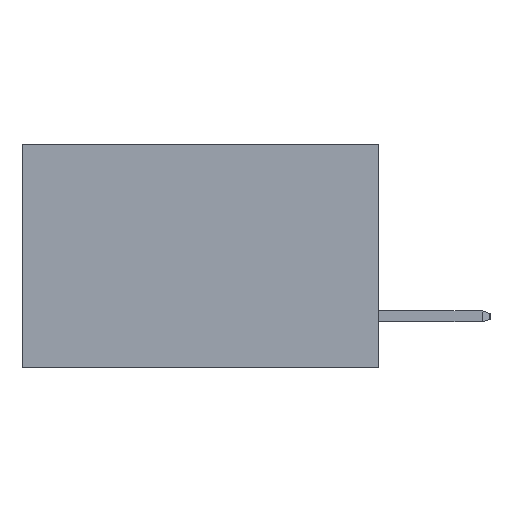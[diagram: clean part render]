
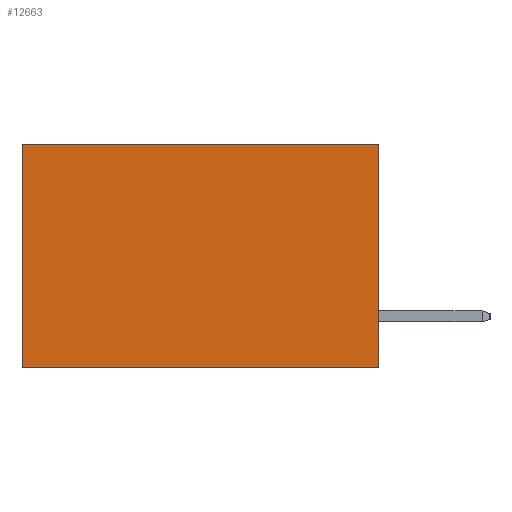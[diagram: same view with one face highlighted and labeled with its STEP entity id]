
A CAD part, left-side view. The second image highlights one B-rep face of the part: STEP entity #12663.
In plain terms, the highlighted planar face has unit normal (-1, 0, 0).
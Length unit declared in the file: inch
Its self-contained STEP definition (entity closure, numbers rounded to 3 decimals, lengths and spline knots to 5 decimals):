
#49 = CARTESIAN_POINT ( 'NONE',  ( 0.277, 0., -0.37 ) ) ;
#526 = LINE ( 'NONE', #4320, #6119 ) ;
#615 = AXIS2_PLACEMENT_3D ( 'NONE', #11861, #12877, #6741 ) ;
#1123 = VERTEX_POINT ( 'NONE', #5369 ) ;
#1202 = VECTOR ( 'NONE', #11866, 39.37008 ) ;
#2030 = DIRECTION ( 'NONE',  ( 0., 0., -1. ) ) ;
#2289 = VECTOR ( 'NONE', #3786, 39.37008 ) ;
#2624 = VERTEX_POINT ( 'NONE', #9195 ) ;
#3365 = VERTEX_POINT ( 'NONE', #5408 ) ;
#3655 = CARTESIAN_POINT ( 'NONE',  ( 0.277, 0.59, -0.37 ) ) ;
#3786 = DIRECTION ( 'NONE',  ( 0., 0., -1. ) ) ;
#4222 = LINE ( 'NONE', #5680, #1202 ) ;
#4320 = CARTESIAN_POINT ( 'NONE',  ( 0.277, 0., -0.37 ) ) ;
#4574 = PLANE ( 'NONE',  #615 ) ;
#4865 = ORIENTED_EDGE ( 'NONE', *, *, #9217, .T. ) ;
#5211 = ORIENTED_EDGE ( 'NONE', *, *, #9500, .F. ) ;
#5369 = CARTESIAN_POINT ( 'NONE',  ( 0.277, 0.59, -0.37 ) ) ;
#5408 = CARTESIAN_POINT ( 'NONE',  ( 0.277, 0.59, 0. ) ) ;
#5680 = CARTESIAN_POINT ( 'NONE',  ( 0.277, 0., 0. ) ) ;
#6119 = VECTOR ( 'NONE', #10634, 39.37008 ) ;
#6741 = DIRECTION ( 'NONE',  ( 0., 0., -1. ) ) ;
#8106 = LINE ( 'NONE', #3655, #2289 ) ;
#8346 = FACE_OUTER_BOUND ( 'NONE', #13686, .T. ) ;
#9195 = CARTESIAN_POINT ( 'NONE',  ( 0.277, 0., -0.37 ) ) ;
#9217 = EDGE_CURVE ( 'NONE', #3365, #1123, #8106, .T. ) ;
#9249 = VECTOR ( 'NONE', #2030, 39.37008 ) ;
#9500 = EDGE_CURVE ( 'NONE', #13172, #2624, #11965, .T. ) ;
#9949 = EDGE_CURVE ( 'NONE', #2624, #1123, #526, .T. ) ;
#10634 = DIRECTION ( 'NONE',  ( 0., 1., 0. ) ) ;
#10659 = EDGE_CURVE ( 'NONE', #13172, #3365, #4222, .T. ) ;
#10762 = ORIENTED_EDGE ( 'NONE', *, *, #10659, .T. ) ;
#11861 = CARTESIAN_POINT ( 'NONE',  ( 0.277, 0., -0.37 ) ) ;
#11866 = DIRECTION ( 'NONE',  ( 0., 1., 0. ) ) ;
#11965 = LINE ( 'NONE', #49, #9249 ) ;
#12663 = ADVANCED_FACE ( 'NONE', ( #8346 ), #4574, .F. ) ;
#12877 = DIRECTION ( 'NONE',  ( 1., 0., 0. ) ) ;
#13132 = ORIENTED_EDGE ( 'NONE', *, *, #9949, .F. ) ;
#13172 = VERTEX_POINT ( 'NONE', #13510 ) ;
#13510 = CARTESIAN_POINT ( 'NONE',  ( 0.277, 0., 0. ) ) ;
#13686 = EDGE_LOOP ( 'NONE', ( #4865, #13132, #5211, #10762 ) ) ;
